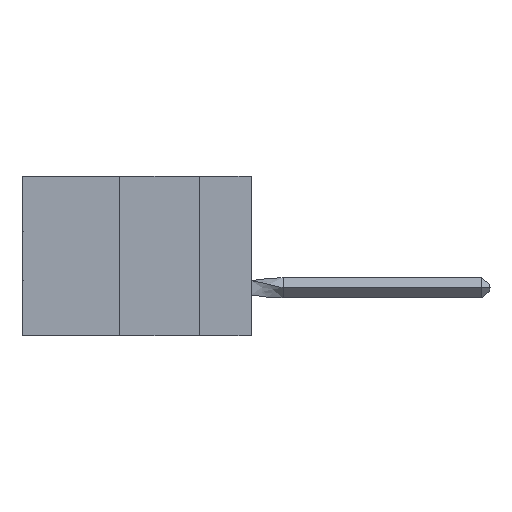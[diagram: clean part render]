
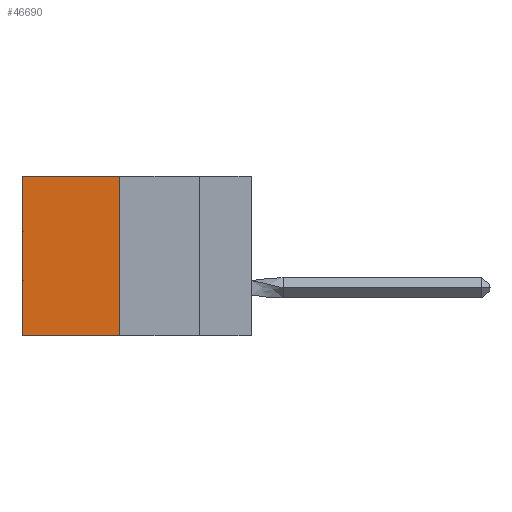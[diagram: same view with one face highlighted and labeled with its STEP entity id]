
A CAD part, left-side view. The second image highlights one B-rep face of the part: STEP entity #46690.
In plain terms, the highlighted planar face has unit normal (-1, 0, 0).
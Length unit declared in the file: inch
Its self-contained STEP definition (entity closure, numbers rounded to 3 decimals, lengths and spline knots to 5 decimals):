
#2322 = DIRECTION ( 'NONE',  ( 0., 0., -1. ) ) ;
#3371 = DIRECTION ( 'NONE',  ( 1., 0., 0. ) ) ;
#3678 = DIRECTION ( 'NONE',  ( 0., 0., -1. ) ) ;
#4462 = AXIS2_PLACEMENT_3D ( 'NONE', #11171, #3371, #3678 ) ;
#6909 = CARTESIAN_POINT ( 'NONE',  ( 0.305, 0.72, -0.5 ) ) ;
#8787 = CARTESIAN_POINT ( 'NONE',  ( 0.305, 0.413, 0. ) ) ;
#11171 = CARTESIAN_POINT ( 'NONE',  ( 0.305, 0.413, -0.5 ) ) ;
#13206 = CARTESIAN_POINT ( 'NONE',  ( 0.305, 0.72, 0. ) ) ;
#14068 = VECTOR ( 'NONE', #18999, 39.37008 ) ;
#14991 = CARTESIAN_POINT ( 'NONE',  ( 0.305, 0.413, 0. ) ) ;
#15421 = PLANE ( 'NONE',  #4462 ) ;
#16212 = VECTOR ( 'NONE', #43114, 39.37008 ) ;
#16455 = LINE ( 'NONE', #39941, #45643 ) ;
#16716 = VERTEX_POINT ( 'NONE', #8787 ) ;
#17142 = EDGE_CURVE ( 'NONE', #16716, #38417, #37932, .T. ) ;
#18999 = DIRECTION ( 'NONE',  ( 0., 1., 0. ) ) ;
#21120 = DIRECTION ( 'NONE',  ( 0., 1., 0. ) ) ;
#22182 = ORIENTED_EDGE ( 'NONE', *, *, #24549, .F. ) ;
#24135 = CARTESIAN_POINT ( 'NONE',  ( 0.305, 0.72, -0.5 ) ) ;
#24549 = EDGE_CURVE ( 'NONE', #37878, #45846, #46289, .T. ) ;
#25650 = EDGE_CURVE ( 'NONE', #16716, #37878, #16455, .T. ) ;
#26324 = LINE ( 'NONE', #24135, #16212 ) ;
#29701 = ORIENTED_EDGE ( 'NONE', *, *, #25650, .F. ) ;
#29857 = ORIENTED_EDGE ( 'NONE', *, *, #48687, .T. ) ;
#32817 = ORIENTED_EDGE ( 'NONE', *, *, #17142, .T. ) ;
#35458 = FACE_OUTER_BOUND ( 'NONE', #48320, .T. ) ;
#36277 = CARTESIAN_POINT ( 'NONE',  ( 0.305, 0.413, -0.5 ) ) ;
#37878 = VERTEX_POINT ( 'NONE', #38053 ) ;
#37932 = LINE ( 'NONE', #14991, #14068 ) ;
#38053 = CARTESIAN_POINT ( 'NONE',  ( 0.305, 0.413, -0.5 ) ) ;
#38417 = VERTEX_POINT ( 'NONE', #13206 ) ;
#39941 = CARTESIAN_POINT ( 'NONE',  ( 0.305, 0.413, -0.5 ) ) ;
#41559 = VECTOR ( 'NONE', #21120, 39.37008 ) ;
#43114 = DIRECTION ( 'NONE',  ( 0., 0., -1. ) ) ;
#45643 = VECTOR ( 'NONE', #2322, 39.37008 ) ;
#45846 = VERTEX_POINT ( 'NONE', #6909 ) ;
#46289 = LINE ( 'NONE', #36277, #41559 ) ;
#46690 = ADVANCED_FACE ( 'NONE', ( #35458 ), #15421, .F. ) ;
#48320 = EDGE_LOOP ( 'NONE', ( #29857, #22182, #29701, #32817 ) ) ;
#48687 = EDGE_CURVE ( 'NONE', #38417, #45846, #26324, .T. ) ;
